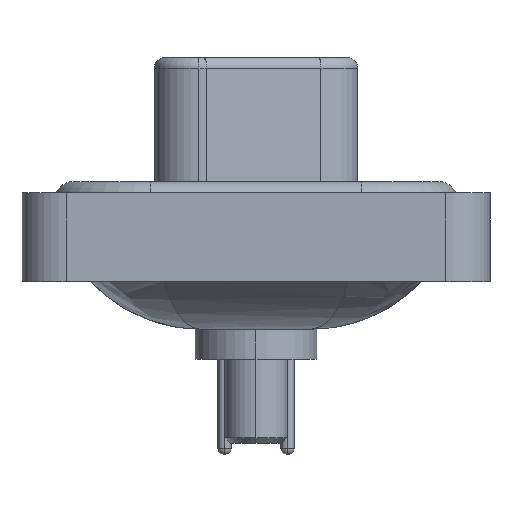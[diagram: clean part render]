
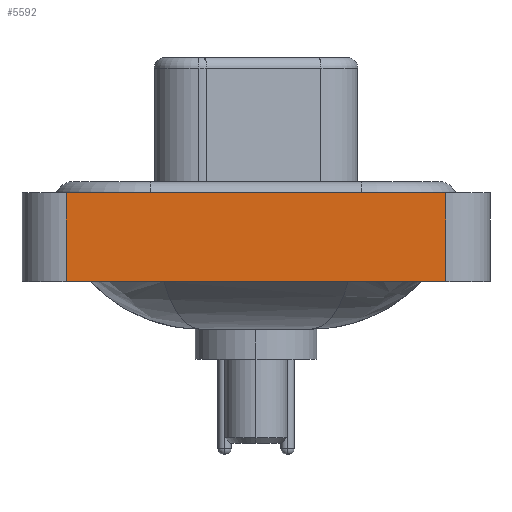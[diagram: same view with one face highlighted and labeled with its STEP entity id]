
A CAD part, left-side view. The second image highlights one B-rep face of the part: STEP entity #5592.
In plain terms, the highlighted planar face has unit normal (-1, 0, 0).
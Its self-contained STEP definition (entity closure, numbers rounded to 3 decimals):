
#696 = VECTOR ( 'NONE', #10059, 1000. ) ;
#802 = CARTESIAN_POINT ( 'NONE',  ( -7.35, -8.55, -3.6 ) ) ;
#1383 = CARTESIAN_POINT ( 'NONE',  ( -7.35, -8.55, 0.4 ) ) ;
#2233 = LINE ( 'NONE', #15447, #19814 ) ;
#2552 = LINE ( 'NONE', #16096, #6178 ) ;
#3806 = DIRECTION ( 'NONE',  ( 0., 0., 1. ) ) ;
#3809 = VECTOR ( 'NONE', #16585, 1000. ) ;
#3962 = EDGE_CURVE ( 'NONE', #14150, #5492, #9618, .T. ) ;
#4676 = EDGE_CURVE ( 'NONE', #17832, #5492, #2552, .T. ) ;
#4795 = ORIENTED_EDGE ( 'NONE', *, *, #4676, .F. ) ;
#5492 = VERTEX_POINT ( 'NONE', #1383 ) ;
#5592 = ADVANCED_FACE ( 'NONE', ( #10740 ), #16228, .T. ) ;
#5885 = CARTESIAN_POINT ( 'NONE',  ( -7.35, 8.55, -3.6 ) ) ;
#6178 = VECTOR ( 'NONE', #19324, 1000. ) ;
#7181 = VERTEX_POINT ( 'NONE', #5885 ) ;
#7823 = DIRECTION ( 'NONE',  ( 0., 0., 1. ) ) ;
#7928 = EDGE_CURVE ( 'NONE', #7181, #17832, #2233, .T. ) ;
#9168 = DIRECTION ( 'NONE',  ( -1., 0., 0. ) ) ;
#9296 = AXIS2_PLACEMENT_3D ( 'NONE', #17584, #9168, #7823 ) ;
#9618 = LINE ( 'NONE', #21956, #3809 ) ;
#10059 = DIRECTION ( 'NONE',  ( 0., -1., 0. ) ) ;
#10740 = FACE_OUTER_BOUND ( 'NONE', #13455, .T. ) ;
#13193 = ORIENTED_EDGE ( 'NONE', *, *, #3962, .T. ) ;
#13455 = EDGE_LOOP ( 'NONE', ( #13193, #4795, #18548, #15201 ) ) ;
#13866 = LINE ( 'NONE', #17115, #696 ) ;
#14150 = VERTEX_POINT ( 'NONE', #802 ) ;
#15201 = ORIENTED_EDGE ( 'NONE', *, *, #22044, .T. ) ;
#15447 = CARTESIAN_POINT ( 'NONE',  ( -7.35, 8.55, -3.6 ) ) ;
#16096 = CARTESIAN_POINT ( 'NONE',  ( -7.35, -8.55, 0.4 ) ) ;
#16228 = PLANE ( 'NONE',  #9296 ) ;
#16585 = DIRECTION ( 'NONE',  ( 0., 0., 1. ) ) ;
#17115 = CARTESIAN_POINT ( 'NONE',  ( -7.35, -8.55, -3.6 ) ) ;
#17584 = CARTESIAN_POINT ( 'NONE',  ( -7.35, -8.55, -3.6 ) ) ;
#17832 = VERTEX_POINT ( 'NONE', #21982 ) ;
#18548 = ORIENTED_EDGE ( 'NONE', *, *, #7928, .F. ) ;
#19324 = DIRECTION ( 'NONE',  ( 0., -1., 0. ) ) ;
#19814 = VECTOR ( 'NONE', #3806, 1000. ) ;
#21956 = CARTESIAN_POINT ( 'NONE',  ( -7.35, -8.55, -3.6 ) ) ;
#21982 = CARTESIAN_POINT ( 'NONE',  ( -7.35, 8.55, 0.4 ) ) ;
#22044 = EDGE_CURVE ( 'NONE', #7181, #14150, #13866, .T. ) ;
